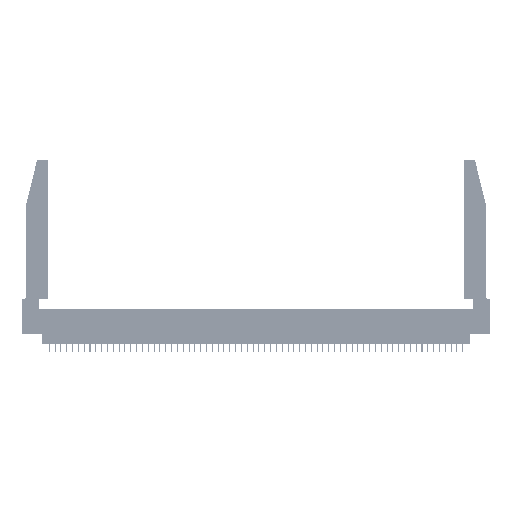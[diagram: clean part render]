
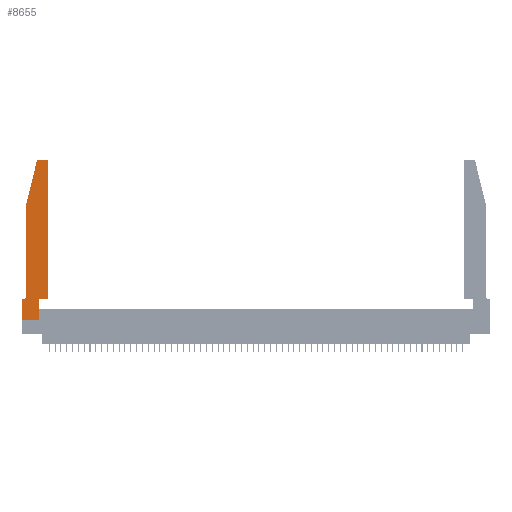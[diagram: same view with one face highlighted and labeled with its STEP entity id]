
A CAD part, top view. The second image highlights one B-rep face of the part: STEP entity #8655.
In plain terms, the highlighted planar face has unit normal (0, 0, 1).
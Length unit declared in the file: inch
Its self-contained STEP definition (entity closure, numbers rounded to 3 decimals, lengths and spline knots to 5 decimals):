
#1111 = CARTESIAN_POINT ( 'NONE',  ( 0.0055, 0.42, 0.37 ) ) ;
#1161 = CARTESIAN_POINT ( 'NONE',  ( 0.284, 2.75, 0.37 ) ) ;
#1927 = CIRCLE ( 'NONE', #45630, 0.03 ) ;
#2175 = VECTOR ( 'NONE', #43384, 39.37008 ) ;
#2826 = ORIENTED_EDGE ( 'NONE', *, *, #44428, .T. ) ;
#2960 = DIRECTION ( 'NONE',  ( 0., -1., 0. ) ) ;
#3103 = VECTOR ( 'NONE', #14165, 39.37008 ) ;
#4244 = CARTESIAN_POINT ( 'NONE',  ( 0., 0., 0.37 ) ) ;
#4940 = VECTOR ( 'NONE', #47580, 39.37008 ) ;
#5073 = DIRECTION ( 'NONE',  ( 1., 0., 0. ) ) ;
#5109 = ORIENTED_EDGE ( 'NONE', *, *, #24280, .T. ) ;
#5142 = CARTESIAN_POINT ( 'NONE',  ( 0., 0., 0.37 ) ) ;
#5378 = ORIENTED_EDGE ( 'NONE', *, *, #31986, .T. ) ;
#5767 = DIRECTION ( 'NONE',  ( 0., 0., -1. ) ) ;
#6327 = ORIENTED_EDGE ( 'NONE', *, *, #39804, .T. ) ;
#6352 = VERTEX_POINT ( 'NONE', #37554 ) ;
#6366 = CARTESIAN_POINT ( 'NONE',  ( 0.0755, 2., 0.37 ) ) ;
#6509 = EDGE_CURVE ( 'NONE', #23388, #51607, #39574, .T. ) ;
#7532 = EDGE_CURVE ( 'NONE', #51607, #34940, #1927, .T. ) ;
#8655 = ADVANCED_FACE ( 'NONE', ( #55420 ), #10949, .T. ) ;
#9514 = VERTEX_POINT ( 'NONE', #28286 ) ;
#9993 = ORIENTED_EDGE ( 'NONE', *, *, #31556, .T. ) ;
#10145 = LINE ( 'NONE', #49122, #48221 ) ;
#10949 = PLANE ( 'NONE',  #47344 ) ;
#14165 = DIRECTION ( 'NONE',  ( 0., -1., 0. ) ) ;
#14827 = EDGE_CURVE ( 'NONE', #42851, #54554, #44989, .T. ) ;
#17294 = VERTEX_POINT ( 'NONE', #24391 ) ;
#17582 = CIRCLE ( 'NONE', #47293, 0.07 ) ;
#18013 = VECTOR ( 'NONE', #30258, 39.37008 ) ;
#18293 = DIRECTION ( 'NONE',  ( 1., 0., 0. ) ) ;
#19335 = EDGE_CURVE ( 'NONE', #54554, #57217, #22879, .T. ) ;
#19511 = CARTESIAN_POINT ( 'NONE',  ( 0., 0., 0.37 ) ) ;
#19723 = VECTOR ( 'NONE', #44297, 39.37008 ) ;
#21911 = CARTESIAN_POINT ( 'NONE',  ( 0.2865, 0., 0.37 ) ) ;
#22010 = DIRECTION ( 'NONE',  ( 1., 0., 0. ) ) ;
#22879 = LINE ( 'NONE', #4244, #38633 ) ;
#23388 = VERTEX_POINT ( 'NONE', #27540 ) ;
#24256 = EDGE_CURVE ( 'NONE', #17294, #54748, #10145, .T. ) ;
#24280 = EDGE_CURVE ( 'NONE', #9514, #6352, #17582, .T. ) ;
#24391 = CARTESIAN_POINT ( 'NONE',  ( 0.2865, 0.35, 0.37 ) ) ;
#24479 = ORIENTED_EDGE ( 'NONE', *, *, #36300, .T. ) ;
#24481 = ORIENTED_EDGE ( 'NONE', *, *, #30536, .T. ) ;
#24621 = DIRECTION ( 'NONE',  ( 1., 0., 0. ) ) ;
#26092 = VERTEX_POINT ( 'NONE', #27272 ) ;
#26278 = LINE ( 'NONE', #31218, #19723 ) ;
#27226 = DIRECTION ( 'NONE',  ( 1., 0., 0. ) ) ;
#27272 = CARTESIAN_POINT ( 'NONE',  ( 0.4505, 2.72, 0.37 ) ) ;
#27540 = CARTESIAN_POINT ( 'NONE',  ( 0.4205, 2.75, 0.37 ) ) ;
#28286 = CARTESIAN_POINT ( 'NONE',  ( 0.0755, 0.42, 0.37 ) ) ;
#30002 = LINE ( 'NONE', #47166, #2175 ) ;
#30258 = DIRECTION ( 'NONE',  ( -1., 0., 0. ) ) ;
#30536 = EDGE_CURVE ( 'NONE', #6352, #42851, #26278, .T. ) ;
#31218 = CARTESIAN_POINT ( 'NONE',  ( 0.0755, 0.35, 0.37 ) ) ;
#31556 = EDGE_CURVE ( 'NONE', #57217, #17294, #34787, .T. ) ;
#31986 = EDGE_CURVE ( 'NONE', #54748, #26092, #43441, .T. ) ;
#32684 = CARTESIAN_POINT ( 'NONE',  ( 0., 0.35, 0.37 ) ) ;
#34210 = DIRECTION ( 'NONE',  ( 0., 0., 1. ) ) ;
#34427 = AXIS2_PLACEMENT_3D ( 'NONE', #35659, #46587, #27226 ) ;
#34787 = LINE ( 'NONE', #38874, #4940 ) ;
#34940 = VERTEX_POINT ( 'NONE', #51252 ) ;
#35197 = CARTESIAN_POINT ( 'NONE',  ( 0.2605, 2.75, 0.37 ) ) ;
#35659 = CARTESIAN_POINT ( 'NONE',  ( 0.4205, 2.72, 0.37 ) ) ;
#36300 = EDGE_CURVE ( 'NONE', #26092, #23388, #52093, .T. ) ;
#36844 = VERTEX_POINT ( 'NONE', #6366 ) ;
#37554 = CARTESIAN_POINT ( 'NONE',  ( 0.0055, 0.35, 0.37 ) ) ;
#37945 = DIRECTION ( 'NONE',  ( 0., 1., 0. ) ) ;
#38342 = VECTOR ( 'NONE', #37945, 39.37008 ) ;
#38633 = VECTOR ( 'NONE', #22010, 39.37008 ) ;
#38874 = CARTESIAN_POINT ( 'NONE',  ( 0.2865, 0.35, 0.37 ) ) ;
#39049 = CARTESIAN_POINT ( 'NONE',  ( 0.0755, 2., 0.37 ) ) ;
#39574 = LINE ( 'NONE', #35197, #18013 ) ;
#39804 = EDGE_CURVE ( 'NONE', #34940, #36844, #30002, .T. ) ;
#42492 = ORIENTED_EDGE ( 'NONE', *, *, #7532, .T. ) ;
#42851 = VERTEX_POINT ( 'NONE', #32684 ) ;
#43384 = DIRECTION ( 'NONE',  ( -0.239, -0.971, 0. ) ) ;
#43403 = LINE ( 'NONE', #39049, #48864 ) ;
#43441 = LINE ( 'NONE', #56531, #38342 ) ;
#44297 = DIRECTION ( 'NONE',  ( -1., 0., 0. ) ) ;
#44428 = EDGE_CURVE ( 'NONE', #36844, #9514, #43403, .T. ) ;
#44989 = LINE ( 'NONE', #5142, #3103 ) ;
#45536 = ORIENTED_EDGE ( 'NONE', *, *, #24256, .T. ) ;
#45630 = AXIS2_PLACEMENT_3D ( 'NONE', #49579, #49284, #5073 ) ;
#45635 = ORIENTED_EDGE ( 'NONE', *, *, #6509, .T. ) ;
#46419 = CARTESIAN_POINT ( 'NONE',  ( 0., 0.35, 0.37 ) ) ;
#46587 = DIRECTION ( 'NONE',  ( 0., 0., 1. ) ) ;
#47166 = CARTESIAN_POINT ( 'NONE',  ( 0.0755, 2., 0.37 ) ) ;
#47293 = AXIS2_PLACEMENT_3D ( 'NONE', #1111, #5767, #54049 ) ;
#47344 = AXIS2_PLACEMENT_3D ( 'NONE', #46419, #34210, #24621 ) ;
#47580 = DIRECTION ( 'NONE',  ( 0., 1., 0. ) ) ;
#48221 = VECTOR ( 'NONE', #18293, 39.37008 ) ;
#48277 = CARTESIAN_POINT ( 'NONE',  ( 0.4505, 0.35, 0.37 ) ) ;
#48864 = VECTOR ( 'NONE', #2960, 39.37008 ) ;
#49122 = CARTESIAN_POINT ( 'NONE',  ( 0.4505, 0.35, 0.37 ) ) ;
#49284 = DIRECTION ( 'NONE',  ( 0., 0., 1. ) ) ;
#49579 = CARTESIAN_POINT ( 'NONE',  ( 0.284, 2.72, 0.37 ) ) ;
#51252 = CARTESIAN_POINT ( 'NONE',  ( 0.25487, 2.72718, 0.37 ) ) ;
#51607 = VERTEX_POINT ( 'NONE', #1161 ) ;
#51765 = EDGE_LOOP ( 'NONE', ( #45635, #42492, #6327, #2826, #5109, #24481, #53985, #54182, #9993, #45536, #5378, #24479 ) ) ;
#52093 = CIRCLE ( 'NONE', #34427, 0.03 ) ;
#53985 = ORIENTED_EDGE ( 'NONE', *, *, #14827, .T. ) ;
#54049 = DIRECTION ( 'NONE',  ( -1., 0., 0. ) ) ;
#54182 = ORIENTED_EDGE ( 'NONE', *, *, #19335, .T. ) ;
#54554 = VERTEX_POINT ( 'NONE', #19511 ) ;
#54748 = VERTEX_POINT ( 'NONE', #48277 ) ;
#55420 = FACE_OUTER_BOUND ( 'NONE', #51765, .T. ) ;
#56531 = CARTESIAN_POINT ( 'NONE',  ( 0.4505, 0.35, 0.37 ) ) ;
#57217 = VERTEX_POINT ( 'NONE', #21911 ) ;
